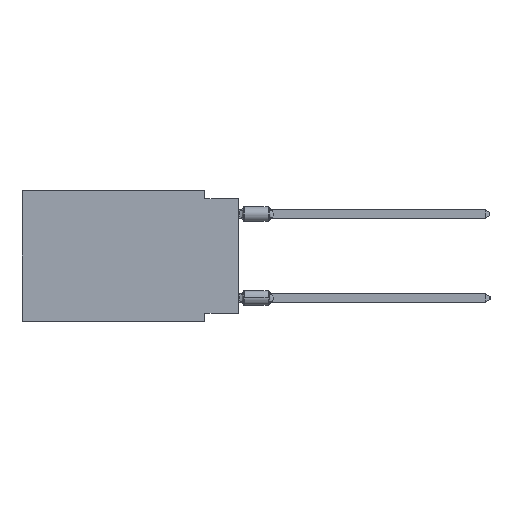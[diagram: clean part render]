
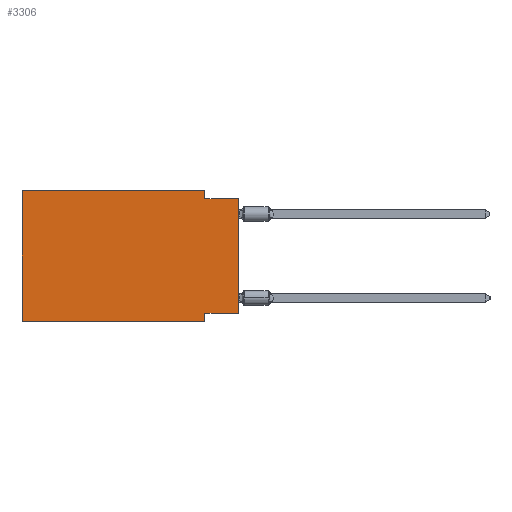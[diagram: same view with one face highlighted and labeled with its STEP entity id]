
A CAD part, left-side view. The second image highlights one B-rep face of the part: STEP entity #3306.
In plain terms, the highlighted planar face has unit normal (-1, 0, 0).
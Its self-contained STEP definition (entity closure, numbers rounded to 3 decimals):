
#942 = DIRECTION ( 'NONE',  ( 0., -1., 0. ) ) ;
#983 = LINE ( 'NONE', #34085, #20721 ) ;
#1954 = ORIENTED_EDGE ( 'NONE', *, *, #25054, .F. ) ;
#1988 = VECTOR ( 'NONE', #34556, 1000. ) ;
#2129 = PLANE ( 'NONE',  #9409 ) ;
#2158 = CARTESIAN_POINT ( 'NONE',  ( 0., 16.383, 0. ) ) ;
#2546 = EDGE_LOOP ( 'NONE', ( #16503, #3880, #7848, #1954, #25970, #16803, #18127, #7885 ) ) ;
#3306 = ADVANCED_FACE ( 'NONE', ( #5530 ), #2129, .F. ) ;
#3665 = VERTEX_POINT ( 'NONE', #15885 ) ;
#3880 = ORIENTED_EDGE ( 'NONE', *, *, #32898, .F. ) ;
#3937 = DIRECTION ( 'NONE',  ( 0., 0., 1. ) ) ;
#5530 = FACE_OUTER_BOUND ( 'NONE', #2546, .T. ) ;
#6262 = DIRECTION ( 'NONE',  ( 0., 0., -1. ) ) ;
#7138 = VECTOR ( 'NONE', #8579, 1000. ) ;
#7848 = ORIENTED_EDGE ( 'NONE', *, *, #13884, .F. ) ;
#7885 = ORIENTED_EDGE ( 'NONE', *, *, #13722, .F. ) ;
#8020 = CARTESIAN_POINT ( 'NONE',  ( 0., 2.54, -9.906 ) ) ;
#8579 = DIRECTION ( 'NONE',  ( 0., 0., -1. ) ) ;
#8974 = CARTESIAN_POINT ( 'NONE',  ( 0., 2.54, 0. ) ) ;
#9115 = CARTESIAN_POINT ( 'NONE',  ( 0., 16.383, 0. ) ) ;
#9409 = AXIS2_PLACEMENT_3D ( 'NONE', #13588, #21465, #10534 ) ;
#9497 = EDGE_CURVE ( 'NONE', #14331, #21208, #17011, .T. ) ;
#10534 = DIRECTION ( 'NONE',  ( 0., 0., -1. ) ) ;
#12904 = CARTESIAN_POINT ( 'NONE',  ( 0., 0., -9.271 ) ) ;
#13401 = CARTESIAN_POINT ( 'NONE',  ( 0., 0., 0. ) ) ;
#13441 = CARTESIAN_POINT ( 'NONE',  ( 0., 2.54, 0. ) ) ;
#13588 = CARTESIAN_POINT ( 'NONE',  ( 0., 16.383, 0. ) ) ;
#13722 = EDGE_CURVE ( 'NONE', #3665, #25788, #26511, .T. ) ;
#13884 = EDGE_CURVE ( 'NONE', #21131, #15483, #22015, .T. ) ;
#14331 = VERTEX_POINT ( 'NONE', #30214 ) ;
#14907 = CARTESIAN_POINT ( 'NONE',  ( 0., 16.383, -9.906 ) ) ;
#15483 = VERTEX_POINT ( 'NONE', #29258 ) ;
#15885 = CARTESIAN_POINT ( 'NONE',  ( 0., 0., -9.271 ) ) ;
#16463 = VECTOR ( 'NONE', #3937, 1000. ) ;
#16503 = ORIENTED_EDGE ( 'NONE', *, *, #16958, .T. ) ;
#16803 = ORIENTED_EDGE ( 'NONE', *, *, #34776, .T. ) ;
#16958 = EDGE_CURVE ( 'NONE', #3665, #26417, #35058, .T. ) ;
#17011 = LINE ( 'NONE', #9115, #16463 ) ;
#17329 = VECTOR ( 'NONE', #18961, 1000. ) ;
#17600 = LINE ( 'NONE', #14907, #27957 ) ;
#18127 = ORIENTED_EDGE ( 'NONE', *, *, #19454, .F. ) ;
#18961 = DIRECTION ( 'NONE',  ( 0., 0., 1. ) ) ;
#19454 = EDGE_CURVE ( 'NONE', #25788, #24139, #30789, .T. ) ;
#19560 = DIRECTION ( 'NONE',  ( 0., -1., 0. ) ) ;
#20721 = VECTOR ( 'NONE', #23180, 1000. ) ;
#20928 = VECTOR ( 'NONE', #19560, 1000. ) ;
#21131 = VERTEX_POINT ( 'NONE', #8974 ) ;
#21208 = VERTEX_POINT ( 'NONE', #2158 ) ;
#21465 = DIRECTION ( 'NONE',  ( 1., 0., 0. ) ) ;
#22015 = LINE ( 'NONE', #13441, #7138 ) ;
#22591 = CARTESIAN_POINT ( 'NONE',  ( 0., 16.383, 0. ) ) ;
#23180 = DIRECTION ( 'NONE',  ( 0., -1., 0. ) ) ;
#24139 = VERTEX_POINT ( 'NONE', #8020 ) ;
#25054 = EDGE_CURVE ( 'NONE', #21208, #21131, #30300, .T. ) ;
#25767 = CARTESIAN_POINT ( 'NONE',  ( 0., 2.54, -9.906 ) ) ;
#25788 = VERTEX_POINT ( 'NONE', #27660 ) ;
#25970 = ORIENTED_EDGE ( 'NONE', *, *, #9497, .F. ) ;
#26417 = VERTEX_POINT ( 'NONE', #31372 ) ;
#26511 = LINE ( 'NONE', #12904, #1988 ) ;
#27660 = CARTESIAN_POINT ( 'NONE',  ( 0., 2.54, -9.271 ) ) ;
#27957 = VECTOR ( 'NONE', #942, 1000. ) ;
#28995 = VECTOR ( 'NONE', #6262, 1000. ) ;
#29258 = CARTESIAN_POINT ( 'NONE',  ( 0., 2.54, -0.635 ) ) ;
#30214 = CARTESIAN_POINT ( 'NONE',  ( 0., 16.383, -9.906 ) ) ;
#30300 = LINE ( 'NONE', #22591, #20928 ) ;
#30789 = LINE ( 'NONE', #25767, #28995 ) ;
#31372 = CARTESIAN_POINT ( 'NONE',  ( 0., 0., -0.635 ) ) ;
#32898 = EDGE_CURVE ( 'NONE', #15483, #26417, #983, .T. ) ;
#34085 = CARTESIAN_POINT ( 'NONE',  ( 0., 0., -0.635 ) ) ;
#34556 = DIRECTION ( 'NONE',  ( 0., 1., 0. ) ) ;
#34776 = EDGE_CURVE ( 'NONE', #14331, #24139, #17600, .T. ) ;
#35058 = LINE ( 'NONE', #13401, #17329 ) ;
